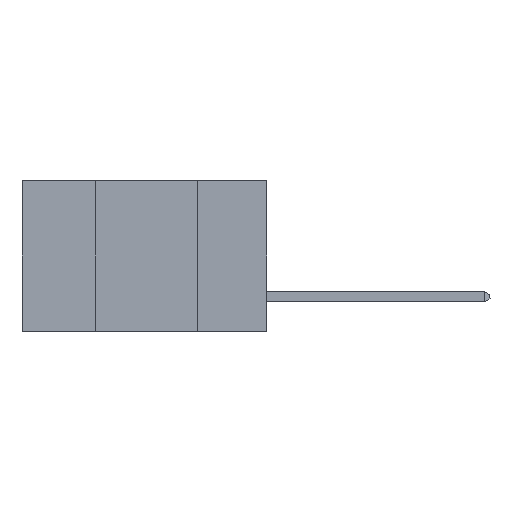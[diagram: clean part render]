
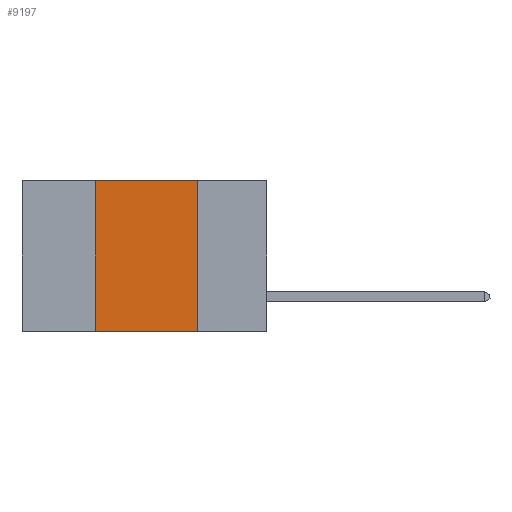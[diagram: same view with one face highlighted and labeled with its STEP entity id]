
A CAD part, left-side view. The second image highlights one B-rep face of the part: STEP entity #9197.
In plain terms, the highlighted planar face has unit normal (-1, 0, 0).
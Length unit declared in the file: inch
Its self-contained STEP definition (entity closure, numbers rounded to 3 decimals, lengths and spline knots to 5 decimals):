
#358 = DIRECTION ( 'NONE',  ( 0., 0., -1. ) ) ;
#1823 = AXIS2_PLACEMENT_3D ( 'NONE', #16624, #8857, #358 ) ;
#2969 = DIRECTION ( 'NONE',  ( 0., 0., 1. ) ) ;
#3386 = VERTEX_POINT ( 'NONE', #13578 ) ;
#3723 = VECTOR ( 'NONE', #16836, 39.37008 ) ;
#4695 = PLANE ( 'NONE',  #1823 ) ;
#4749 = CARTESIAN_POINT ( 'NONE',  ( 0., 0.42, 0. ) ) ;
#5827 = EDGE_CURVE ( 'NONE', #3386, #5908, #11193, .T. ) ;
#5908 = VERTEX_POINT ( 'NONE', #10852 ) ;
#5961 = EDGE_LOOP ( 'NONE', ( #9247, #6750, #13624, #8446 ) ) ;
#6299 = VERTEX_POINT ( 'NONE', #4749 ) ;
#6692 = DIRECTION ( 'NONE',  ( 0., 0., -1. ) ) ;
#6750 = ORIENTED_EDGE ( 'NONE', *, *, #6783, .F. ) ;
#6783 = EDGE_CURVE ( 'NONE', #6299, #3386, #7197, .T. ) ;
#7197 = LINE ( 'NONE', #17530, #10346 ) ;
#8097 = VERTEX_POINT ( 'NONE', #12451 ) ;
#8446 = ORIENTED_EDGE ( 'NONE', *, *, #11011, .T. ) ;
#8480 = DIRECTION ( 'NONE',  ( 0., -1., 0. ) ) ;
#8539 = CARTESIAN_POINT ( 'NONE',  ( 0., 0.42, 0. ) ) ;
#8857 = DIRECTION ( 'NONE',  ( 1., 0., 0. ) ) ;
#9197 = ADVANCED_FACE ( 'NONE', ( #14086 ), #4695, .F. ) ;
#9247 = ORIENTED_EDGE ( 'NONE', *, *, #5827, .F. ) ;
#10132 = EDGE_CURVE ( 'NONE', #8097, #6299, #16076, .T. ) ;
#10346 = VECTOR ( 'NONE', #8480, 39.37008 ) ;
#10735 = CARTESIAN_POINT ( 'NONE',  ( 0., 0.17, 0. ) ) ;
#10852 = CARTESIAN_POINT ( 'NONE',  ( 0., 0.17, -0.37 ) ) ;
#11011 = EDGE_CURVE ( 'NONE', #8097, #5908, #14400, .T. ) ;
#11193 = LINE ( 'NONE', #10735, #11985 ) ;
#11985 = VECTOR ( 'NONE', #6692, 39.37008 ) ;
#12451 = CARTESIAN_POINT ( 'NONE',  ( 0., 0.42, -0.37 ) ) ;
#13578 = CARTESIAN_POINT ( 'NONE',  ( 0., 0.17, 0. ) ) ;
#13624 = ORIENTED_EDGE ( 'NONE', *, *, #10132, .F. ) ;
#14086 = FACE_OUTER_BOUND ( 'NONE', #5961, .T. ) ;
#14400 = LINE ( 'NONE', #15550, #3723 ) ;
#15550 = CARTESIAN_POINT ( 'NONE',  ( 0., 0.6, -0.37 ) ) ;
#15671 = VECTOR ( 'NONE', #2969, 39.37008 ) ;
#16076 = LINE ( 'NONE', #8539, #15671 ) ;
#16624 = CARTESIAN_POINT ( 'NONE',  ( 0., 0.6, 0. ) ) ;
#16836 = DIRECTION ( 'NONE',  ( 0., -1., 0. ) ) ;
#17530 = CARTESIAN_POINT ( 'NONE',  ( 0., 0.6, 0. ) ) ;
